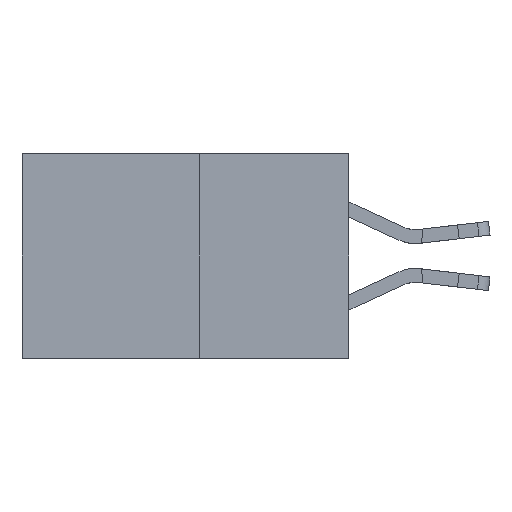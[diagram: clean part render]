
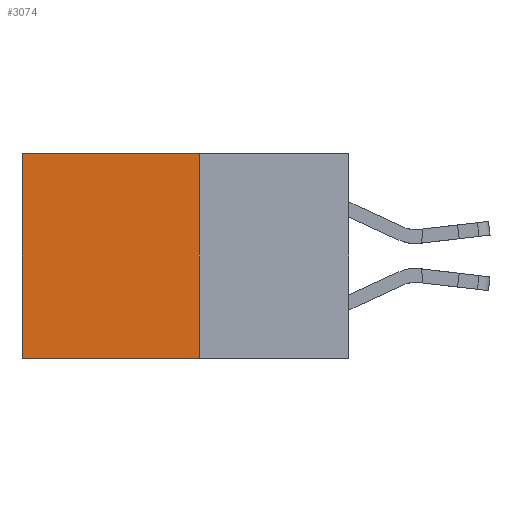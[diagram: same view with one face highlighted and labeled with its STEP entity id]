
A CAD part, left-side view. The second image highlights one B-rep face of the part: STEP entity #3074.
In plain terms, the highlighted planar face has unit normal (-1, 0, 0).
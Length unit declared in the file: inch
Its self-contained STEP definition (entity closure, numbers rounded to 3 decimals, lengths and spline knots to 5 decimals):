
#453 = LINE ( 'NONE', #4695, #17974 ) ;
#778 = LINE ( 'NONE', #20036, #13333 ) ;
#1603 = VERTEX_POINT ( 'NONE', #17693 ) ;
#3074 = ADVANCED_FACE ( 'NONE', ( #19947 ), #16145, .F. ) ;
#3316 = VECTOR ( 'NONE', #21640, 39.37008 ) ;
#3614 = VERTEX_POINT ( 'NONE', #18234 ) ;
#3803 = DIRECTION ( 'NONE',  ( 0., 0., -1. ) ) ;
#4675 = ORIENTED_EDGE ( 'NONE', *, *, #18252, .T. ) ;
#4695 = CARTESIAN_POINT ( 'NONE',  ( 0.277, 0.59, -0.37 ) ) ;
#5939 = EDGE_CURVE ( 'NONE', #9434, #7552, #8685, .T. ) ;
#6101 = ORIENTED_EDGE ( 'NONE', *, *, #16014, .T. ) ;
#6553 = DIRECTION ( 'NONE',  ( 0., 1., 0. ) ) ;
#7552 = VERTEX_POINT ( 'NONE', #19759 ) ;
#8627 = ORIENTED_EDGE ( 'NONE', *, *, #19609, .F. ) ;
#8685 = LINE ( 'NONE', #14053, #13240 ) ;
#9434 = VERTEX_POINT ( 'NONE', #14274 ) ;
#11591 = DIRECTION ( 'NONE',  ( 0., 0., -1. ) ) ;
#13240 = VECTOR ( 'NONE', #3803, 39.37008 ) ;
#13333 = VECTOR ( 'NONE', #6553, 39.37008 ) ;
#13477 = LINE ( 'NONE', #13478, #3316 ) ;
#13478 = CARTESIAN_POINT ( 'NONE',  ( 0.277, 0.27, -0.37 ) ) ;
#14053 = CARTESIAN_POINT ( 'NONE',  ( 0.277, 0.27, -0.37 ) ) ;
#14274 = CARTESIAN_POINT ( 'NONE',  ( 0.277, 0.27, 0. ) ) ;
#15508 = DIRECTION ( 'NONE',  ( 0., 0., -1. ) ) ;
#15578 = DIRECTION ( 'NONE',  ( 1., 0., 0. ) ) ;
#15860 = CARTESIAN_POINT ( 'NONE',  ( 0.277, 0.27, -0.37 ) ) ;
#16014 = EDGE_CURVE ( 'NONE', #9434, #3614, #778, .T. ) ;
#16145 = PLANE ( 'NONE',  #18975 ) ;
#17693 = CARTESIAN_POINT ( 'NONE',  ( 0.277, 0.59, -0.37 ) ) ;
#17974 = VECTOR ( 'NONE', #11591, 39.37008 ) ;
#18234 = CARTESIAN_POINT ( 'NONE',  ( 0.277, 0.59, 0. ) ) ;
#18252 = EDGE_CURVE ( 'NONE', #3614, #1603, #453, .T. ) ;
#18975 = AXIS2_PLACEMENT_3D ( 'NONE', #15860, #15578, #15508 ) ;
#19609 = EDGE_CURVE ( 'NONE', #7552, #1603, #13477, .T. ) ;
#19759 = CARTESIAN_POINT ( 'NONE',  ( 0.277, 0.27, -0.37 ) ) ;
#19947 = FACE_OUTER_BOUND ( 'NONE', #21212, .T. ) ;
#20036 = CARTESIAN_POINT ( 'NONE',  ( 0.277, 0.27, 0. ) ) ;
#20398 = ORIENTED_EDGE ( 'NONE', *, *, #5939, .F. ) ;
#21212 = EDGE_LOOP ( 'NONE', ( #4675, #8627, #20398, #6101 ) ) ;
#21640 = DIRECTION ( 'NONE',  ( 0., 1., 0. ) ) ;
